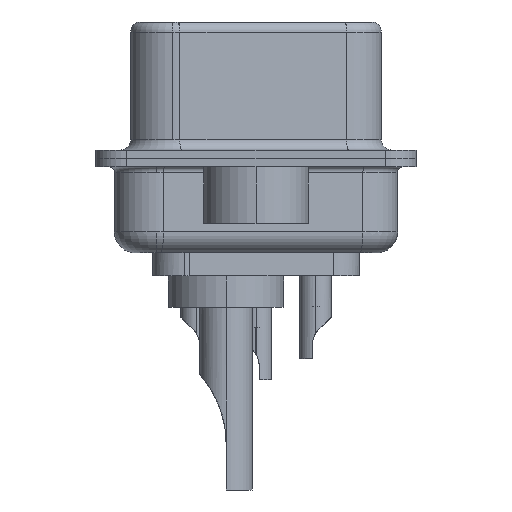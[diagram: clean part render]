
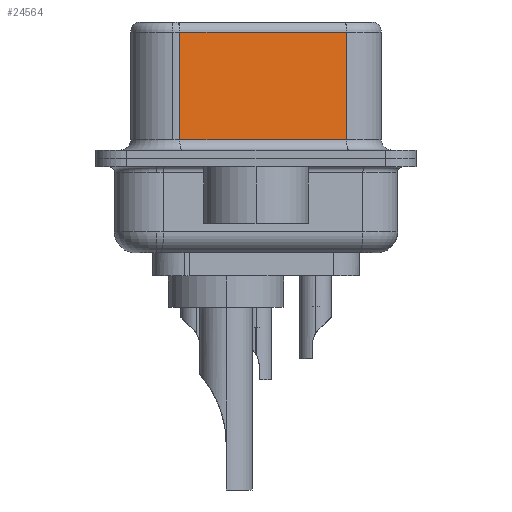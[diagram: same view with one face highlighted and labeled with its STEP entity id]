
A CAD part, left-side view. The second image highlights one B-rep face of the part: STEP entity #24564.
In plain terms, the highlighted planar face has unit normal (-0.985, -0.174, 0).
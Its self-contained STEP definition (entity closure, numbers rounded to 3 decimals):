
#264 = VERTEX_POINT ( 'NONE', #13770 ) ;
#807 = CARTESIAN_POINT ( 'NONE',  ( 5.132, -4.322, 0.9 ) ) ;
#874 = LINE ( 'NONE', #1129, #12338 ) ;
#1129 = CARTESIAN_POINT ( 'NONE',  ( 5.132, -4.322, 6.52 ) ) ;
#1334 = DIRECTION ( 'NONE',  ( -0.174, 0.985, 0. ) ) ;
#2036 = LINE ( 'NONE', #25942, #17629 ) ;
#2511 = DIRECTION ( 'NONE',  ( 0., 0., -1. ) ) ;
#3474 = DIRECTION ( 'NONE',  ( -0.174, 0.985, 0. ) ) ;
#4371 = ORIENTED_EDGE ( 'NONE', *, *, #13162, .T. ) ;
#4565 = CARTESIAN_POINT ( 'NONE',  ( 3.73, 3.628, 6.52 ) ) ;
#4987 = DIRECTION ( 'NONE',  ( 0.174, -0.985, 0. ) ) ;
#5274 = ORIENTED_EDGE ( 'NONE', *, *, #17424, .T. ) ;
#9782 = LINE ( 'NONE', #807, #20047 ) ;
#10815 = EDGE_CURVE ( 'NONE', #23281, #264, #874, .T. ) ;
#12338 = VECTOR ( 'NONE', #15383, 1000. ) ;
#12912 = LINE ( 'NONE', #4565, #22615 ) ;
#13050 = EDGE_CURVE ( 'NONE', #16140, #25892, #12912, .T. ) ;
#13162 = EDGE_CURVE ( 'NONE', #25892, #264, #9782, .T. ) ;
#13770 = CARTESIAN_POINT ( 'NONE',  ( 5.132, -4.322, 0.9 ) ) ;
#14883 = FACE_OUTER_BOUND ( 'NONE', #15847, .T. ) ;
#15383 = DIRECTION ( 'NONE',  ( 0., 0., -1. ) ) ;
#15630 = DIRECTION ( 'NONE',  ( 0.985, 0.174, 0. ) ) ;
#15847 = EDGE_LOOP ( 'NONE', ( #22759, #5274, #22027, #4371 ) ) ;
#16140 = VERTEX_POINT ( 'NONE', #23864 ) ;
#17424 = EDGE_CURVE ( 'NONE', #23281, #16140, #2036, .T. ) ;
#17629 = VECTOR ( 'NONE', #1334, 1000. ) ;
#19727 = CARTESIAN_POINT ( 'NONE',  ( 5.132, -4.322, 6.52 ) ) ;
#19951 = AXIS2_PLACEMENT_3D ( 'NONE', #19727, #15630, #3474 ) ;
#20047 = VECTOR ( 'NONE', #4987, 1000. ) ;
#21943 = CARTESIAN_POINT ( 'NONE',  ( 3.73, 3.628, 0.9 ) ) ;
#22027 = ORIENTED_EDGE ( 'NONE', *, *, #13050, .T. ) ;
#22615 = VECTOR ( 'NONE', #2511, 1000. ) ;
#22759 = ORIENTED_EDGE ( 'NONE', *, *, #10815, .F. ) ;
#23281 = VERTEX_POINT ( 'NONE', #25694 ) ;
#23847 = PLANE ( 'NONE',  #19951 ) ;
#23864 = CARTESIAN_POINT ( 'NONE',  ( 3.73, 3.628, 6.02 ) ) ;
#24564 = ADVANCED_FACE ( 'NONE', ( #14883 ), #23847, .F. ) ;
#25694 = CARTESIAN_POINT ( 'NONE',  ( 5.132, -4.322, 6.02 ) ) ;
#25892 = VERTEX_POINT ( 'NONE', #21943 ) ;
#25942 = CARTESIAN_POINT ( 'NONE',  ( 5.132, -4.322, 6.02 ) ) ;
